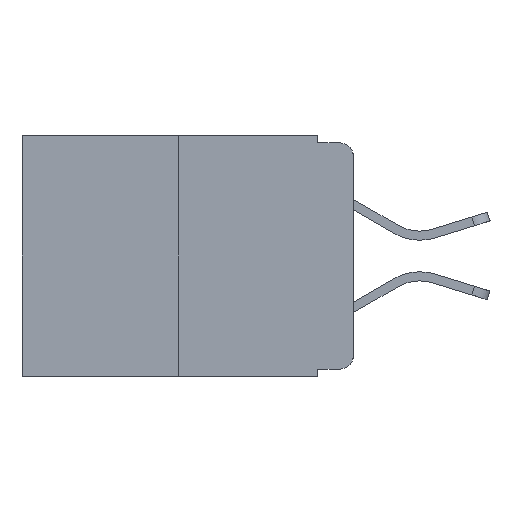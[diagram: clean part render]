
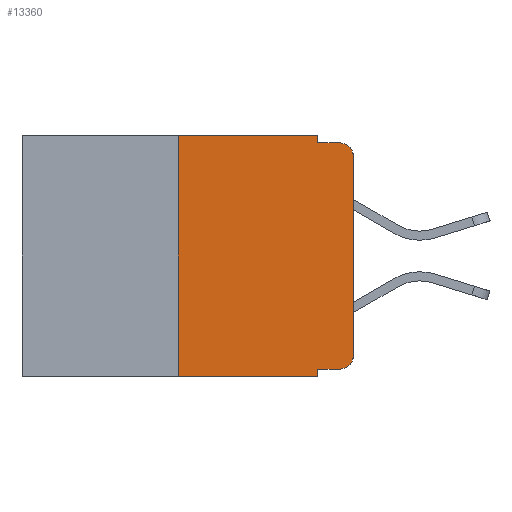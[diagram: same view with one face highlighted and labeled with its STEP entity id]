
A CAD part, left-side view. The second image highlights one B-rep face of the part: STEP entity #13360.
In plain terms, the highlighted planar face has unit normal (-1, 0, 0).
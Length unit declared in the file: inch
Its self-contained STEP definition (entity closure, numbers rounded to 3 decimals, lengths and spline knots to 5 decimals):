
#124 = VECTOR ( 'NONE', #17793, 39.37008 ) ;
#245 = LINE ( 'NONE', #17878, #14963 ) ;
#600 = ORIENTED_EDGE ( 'NONE', *, *, #4569, .T. ) ;
#623 = ORIENTED_EDGE ( 'NONE', *, *, #2682, .T. ) ;
#1301 = DIRECTION ( 'NONE',  ( 0., 0., 1. ) ) ;
#1618 = VECTOR ( 'NONE', #3530, 39.37008 ) ;
#2367 = CARTESIAN_POINT ( 'NONE',  ( 0., 0., -0.313 ) ) ;
#2418 = EDGE_CURVE ( 'NONE', #8577, #4953, #7160, .T. ) ;
#2534 = ORIENTED_EDGE ( 'NONE', *, *, #2418, .F. ) ;
#2595 = CIRCLE ( 'NONE', #6137, 0.02 ) ;
#2682 = EDGE_CURVE ( 'NONE', #5336, #15662, #14813, .T. ) ;
#2941 = CARTESIAN_POINT ( 'NONE',  ( 0., 0.25, -0.343 ) ) ;
#3530 = DIRECTION ( 'NONE',  ( 0., 0., 1. ) ) ;
#3678 = VECTOR ( 'NONE', #16263, 39.37008 ) ;
#3797 = VERTEX_POINT ( 'NONE', #21077 ) ;
#3836 = CARTESIAN_POINT ( 'NONE',  ( 0., 0.02, -0.01 ) ) ;
#3843 = VERTEX_POINT ( 'NONE', #21146 ) ;
#4052 = CARTESIAN_POINT ( 'NONE',  ( 0., 0.25, 0. ) ) ;
#4261 = CARTESIAN_POINT ( 'NONE',  ( 0., 0.051, -0.333 ) ) ;
#4284 = DIRECTION ( 'NONE',  ( 0., 0., -1. ) ) ;
#4434 = EDGE_CURVE ( 'NONE', #6026, #3797, #5306, .T. ) ;
#4445 = CARTESIAN_POINT ( 'NONE',  ( 0., 0.051, 0. ) ) ;
#4569 = EDGE_CURVE ( 'NONE', #18768, #18946, #2595, .T. ) ;
#4705 = ORIENTED_EDGE ( 'NONE', *, *, #6597, .F. ) ;
#4807 = DIRECTION ( 'NONE',  ( -1., 0., 0. ) ) ;
#4953 = VERTEX_POINT ( 'NONE', #4052 ) ;
#5028 = CARTESIAN_POINT ( 'NONE',  ( 0., 0.02, -0.333 ) ) ;
#5306 = LINE ( 'NONE', #4445, #124 ) ;
#5336 = VERTEX_POINT ( 'NONE', #8605 ) ;
#6026 = VERTEX_POINT ( 'NONE', #14007 ) ;
#6137 = AXIS2_PLACEMENT_3D ( 'NONE', #14939, #4807, #16590 ) ;
#6597 = EDGE_CURVE ( 'NONE', #3843, #16395, #15268, .T. ) ;
#6799 = ORIENTED_EDGE ( 'NONE', *, *, #21302, .T. ) ;
#7160 = LINE ( 'NONE', #13960, #10654 ) ;
#7494 = DIRECTION ( 'NONE',  ( 0., 0., -1. ) ) ;
#7545 = AXIS2_PLACEMENT_3D ( 'NONE', #19923, #21138, #4284 ) ;
#7554 = EDGE_CURVE ( 'NONE', #18946, #5336, #19541, .T. ) ;
#7903 = CARTESIAN_POINT ( 'NONE',  ( 0., 0.051, 0. ) ) ;
#8577 = VERTEX_POINT ( 'NONE', #2941 ) ;
#8605 = CARTESIAN_POINT ( 'NONE',  ( 0., 0., -0.03 ) ) ;
#9624 = DIRECTION ( 'NONE',  ( 0., -1., 0. ) ) ;
#9645 = DIRECTION ( 'NONE',  ( 0., 0., -1. ) ) ;
#10654 = VECTOR ( 'NONE', #1301, 39.37008 ) ;
#10830 = VECTOR ( 'NONE', #9645, 39.37008 ) ;
#10895 = CARTESIAN_POINT ( 'NONE',  ( 0., 0.051, -0.01 ) ) ;
#11441 = VECTOR ( 'NONE', #18532, 39.37008 ) ;
#11660 = FACE_OUTER_BOUND ( 'NONE', #19837, .T. ) ;
#12475 = LINE ( 'NONE', #16905, #11441 ) ;
#12843 = EDGE_CURVE ( 'NONE', #8577, #3797, #20905, .T. ) ;
#13360 = ADVANCED_FACE ( 'NONE', ( #11660 ), #15873, .F. ) ;
#13736 = ORIENTED_EDGE ( 'NONE', *, *, #4434, .F. ) ;
#13960 = CARTESIAN_POINT ( 'NONE',  ( 0., 0.25, 0. ) ) ;
#14007 = CARTESIAN_POINT ( 'NONE',  ( 0., 0.051, -0.333 ) ) ;
#14231 = VECTOR ( 'NONE', #19310, 39.37008 ) ;
#14281 = AXIS2_PLACEMENT_3D ( 'NONE', #15802, #17515, #7494 ) ;
#14813 = CIRCLE ( 'NONE', #7545, 0.02 ) ;
#14939 = CARTESIAN_POINT ( 'NONE',  ( 0., 0.02, -0.313 ) ) ;
#14963 = VECTOR ( 'NONE', #9624, 39.37008 ) ;
#15245 = EDGE_CURVE ( 'NONE', #4953, #3843, #245, .T. ) ;
#15268 = LINE ( 'NONE', #7903, #10830 ) ;
#15662 = VERTEX_POINT ( 'NONE', #3836 ) ;
#15802 = CARTESIAN_POINT ( 'NONE',  ( 0., 0.473, 0. ) ) ;
#15873 = PLANE ( 'NONE',  #14281 ) ;
#16016 = ORIENTED_EDGE ( 'NONE', *, *, #19972, .F. ) ;
#16263 = DIRECTION ( 'NONE',  ( 0., -1., 0. ) ) ;
#16395 = VERTEX_POINT ( 'NONE', #10895 ) ;
#16590 = DIRECTION ( 'NONE',  ( 0., 0., -1. ) ) ;
#16905 = CARTESIAN_POINT ( 'NONE',  ( 0., 0.051, -0.01 ) ) ;
#17021 = CARTESIAN_POINT ( 'NONE',  ( 0., 0., 0. ) ) ;
#17515 = DIRECTION ( 'NONE',  ( 1., 0., 0. ) ) ;
#17793 = DIRECTION ( 'NONE',  ( 0., 0., -1. ) ) ;
#17878 = CARTESIAN_POINT ( 'NONE',  ( 0., 0.473, 0. ) ) ;
#18532 = DIRECTION ( 'NONE',  ( 0., -1., 0. ) ) ;
#18586 = LINE ( 'NONE', #4261, #14231 ) ;
#18768 = VERTEX_POINT ( 'NONE', #5028 ) ;
#18946 = VERTEX_POINT ( 'NONE', #2367 ) ;
#19310 = DIRECTION ( 'NONE',  ( 0., -1., 0. ) ) ;
#19519 = CARTESIAN_POINT ( 'NONE',  ( 0., 0.473, -0.343 ) ) ;
#19541 = LINE ( 'NONE', #17021, #1618 ) ;
#19825 = ORIENTED_EDGE ( 'NONE', *, *, #12843, .T. ) ;
#19837 = EDGE_LOOP ( 'NONE', ( #21407, #623, #16016, #4705, #20342, #2534, #19825, #13736, #6799, #600 ) ) ;
#19923 = CARTESIAN_POINT ( 'NONE',  ( 0., 0.02, -0.03 ) ) ;
#19972 = EDGE_CURVE ( 'NONE', #16395, #15662, #12475, .T. ) ;
#20342 = ORIENTED_EDGE ( 'NONE', *, *, #15245, .F. ) ;
#20905 = LINE ( 'NONE', #19519, #3678 ) ;
#21077 = CARTESIAN_POINT ( 'NONE',  ( 0., 0.051, -0.343 ) ) ;
#21138 = DIRECTION ( 'NONE',  ( -1., 0., 0. ) ) ;
#21146 = CARTESIAN_POINT ( 'NONE',  ( 0., 0.051, 0. ) ) ;
#21302 = EDGE_CURVE ( 'NONE', #6026, #18768, #18586, .T. ) ;
#21407 = ORIENTED_EDGE ( 'NONE', *, *, #7554, .T. ) ;
